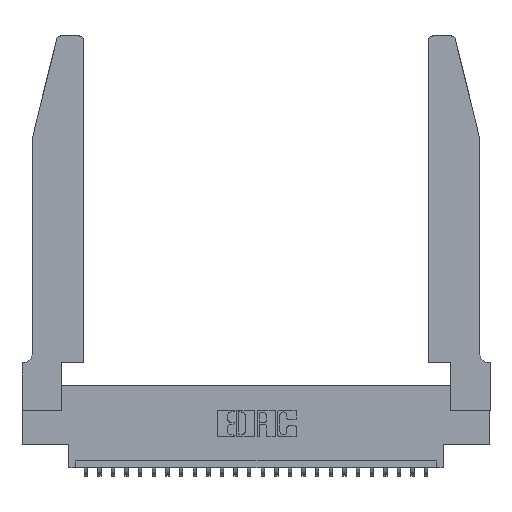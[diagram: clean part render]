
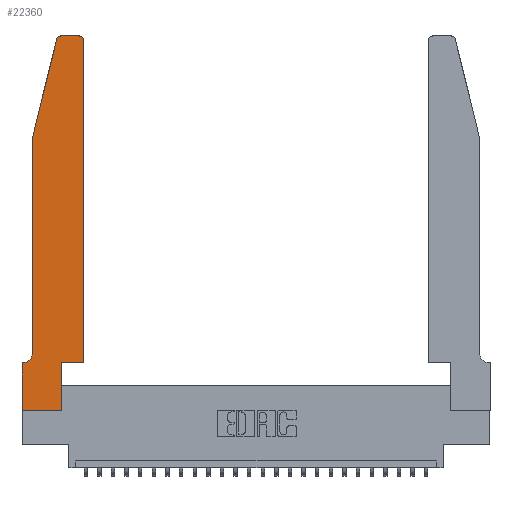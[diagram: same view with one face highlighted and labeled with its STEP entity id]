
A CAD part, top view. The second image highlights one B-rep face of the part: STEP entity #22360.
In plain terms, the highlighted planar face has unit normal (0, 0, 1).
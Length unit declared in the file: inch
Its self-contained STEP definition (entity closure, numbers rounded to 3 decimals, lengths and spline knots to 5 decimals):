
#318 = VERTEX_POINT ( 'NONE', #5157 ) ;
#480 = EDGE_CURVE ( 'NONE', #1135, #4920, #22333, .T. ) ;
#622 = DIRECTION ( 'NONE',  ( 0., 0., 1. ) ) ;
#647 = DIRECTION ( 'NONE',  ( 1., 0., 0. ) ) ;
#790 = VERTEX_POINT ( 'NONE', #2630 ) ;
#998 = VERTEX_POINT ( 'NONE', #18173 ) ;
#1016 = CIRCLE ( 'NONE', #6635, 0.07 ) ;
#1135 = VERTEX_POINT ( 'NONE', #14024 ) ;
#1157 = CARTESIAN_POINT ( 'NONE',  ( 0.0755, 2., 0.37 ) ) ;
#1340 = CARTESIAN_POINT ( 'NONE',  ( 0., 0., 0.37 ) ) ;
#2153 = LINE ( 'NONE', #1157, #8272 ) ;
#2320 = CARTESIAN_POINT ( 'NONE',  ( 0.4505, 0.35, 0.37 ) ) ;
#2576 = VECTOR ( 'NONE', #7749, 39.37008 ) ;
#2629 = LINE ( 'NONE', #14232, #23256 ) ;
#2630 = CARTESIAN_POINT ( 'NONE',  ( 0.0755, 0.42, 0.37 ) ) ;
#3535 = DIRECTION ( 'NONE',  ( 1., 0., 0. ) ) ;
#3636 = CARTESIAN_POINT ( 'NONE',  ( 0.2865, 0.35, 0.37 ) ) ;
#4067 = CARTESIAN_POINT ( 'NONE',  ( 0.0755, 2., 0.37 ) ) ;
#4335 = CARTESIAN_POINT ( 'NONE',  ( 0.2865, 0.35, 0.37 ) ) ;
#4726 = AXIS2_PLACEMENT_3D ( 'NONE', #23396, #622, #15299 ) ;
#4920 = VERTEX_POINT ( 'NONE', #17400 ) ;
#4993 = AXIS2_PLACEMENT_3D ( 'NONE', #7697, #9684, #3535 ) ;
#5065 = CARTESIAN_POINT ( 'NONE',  ( 0.0755, 2., 0.37 ) ) ;
#5157 = CARTESIAN_POINT ( 'NONE',  ( 0.284, 2.75, 0.37 ) ) ;
#5229 = EDGE_CURVE ( 'NONE', #998, #10294, #14947, .T. ) ;
#5653 = CARTESIAN_POINT ( 'NONE',  ( 0.2605, 2.75, 0.37 ) ) ;
#5878 = VERTEX_POINT ( 'NONE', #10979 ) ;
#6230 = AXIS2_PLACEMENT_3D ( 'NONE', #15417, #9199, #647 ) ;
#6256 = DIRECTION ( 'NONE',  ( 0., 1., 0. ) ) ;
#6635 = AXIS2_PLACEMENT_3D ( 'NONE', #18377, #10430, #12156 ) ;
#7697 = CARTESIAN_POINT ( 'NONE',  ( 0.4205, 2.72, 0.37 ) ) ;
#7749 = DIRECTION ( 'NONE',  ( -1., 0., 0. ) ) ;
#8272 = VECTOR ( 'NONE', #19018, 39.37008 ) ;
#8887 = CARTESIAN_POINT ( 'NONE',  ( 0.4505, 0.35, 0.37 ) ) ;
#8955 = VECTOR ( 'NONE', #6256, 39.37008 ) ;
#8995 = VECTOR ( 'NONE', #10202, 39.37008 ) ;
#9176 = PLANE ( 'NONE',  #4726 ) ;
#9195 = ORIENTED_EDGE ( 'NONE', *, *, #9558, .T. ) ;
#9199 = DIRECTION ( 'NONE',  ( 0., 0., 1. ) ) ;
#9322 = EDGE_CURVE ( 'NONE', #24941, #790, #2153, .T. ) ;
#9558 = EDGE_CURVE ( 'NONE', #9641, #13519, #26022, .T. ) ;
#9584 = ORIENTED_EDGE ( 'NONE', *, *, #480, .T. ) ;
#9641 = VERTEX_POINT ( 'NONE', #8887 ) ;
#9684 = DIRECTION ( 'NONE',  ( 0., 0., 1. ) ) ;
#9736 = ORIENTED_EDGE ( 'NONE', *, *, #17080, .T. ) ;
#9824 = VERTEX_POINT ( 'NONE', #13963 ) ;
#10073 = VERTEX_POINT ( 'NONE', #24346 ) ;
#10202 = DIRECTION ( 'NONE',  ( -0.239, -0.971, 0. ) ) ;
#10294 = VERTEX_POINT ( 'NONE', #4335 ) ;
#10430 = DIRECTION ( 'NONE',  ( 0., 0., -1. ) ) ;
#10976 = ORIENTED_EDGE ( 'NONE', *, *, #9322, .T. ) ;
#10979 = CARTESIAN_POINT ( 'NONE',  ( 0.4205, 2.75, 0.37 ) ) ;
#11011 = EDGE_CURVE ( 'NONE', #318, #10073, #23031, .T. ) ;
#11467 = DIRECTION ( 'NONE',  ( -1., 0., 0. ) ) ;
#11927 = DIRECTION ( 'NONE',  ( 0., 1., 0. ) ) ;
#12156 = DIRECTION ( 'NONE',  ( -1., 0., 0. ) ) ;
#12708 = EDGE_LOOP ( 'NONE', ( #9736, #14840, #15039, #10976, #24352, #9584, #16320, #15497, #25948, #16778, #9195, #26026 ) ) ;
#13519 = VERTEX_POINT ( 'NONE', #24000 ) ;
#13668 = LINE ( 'NONE', #1340, #15914 ) ;
#13963 = CARTESIAN_POINT ( 'NONE',  ( 0., 0., 0.37 ) ) ;
#14024 = CARTESIAN_POINT ( 'NONE',  ( 0.0055, 0.35, 0.37 ) ) ;
#14232 = CARTESIAN_POINT ( 'NONE',  ( 0.4505, 0.35, 0.37 ) ) ;
#14840 = ORIENTED_EDGE ( 'NONE', *, *, #11011, .T. ) ;
#14947 = LINE ( 'NONE', #3636, #19771 ) ;
#15039 = ORIENTED_EDGE ( 'NONE', *, *, #23353, .T. ) ;
#15143 = LINE ( 'NONE', #5653, #2576 ) ;
#15299 = DIRECTION ( 'NONE',  ( 1., 0., 0. ) ) ;
#15417 = CARTESIAN_POINT ( 'NONE',  ( 0.284, 2.72, 0.37 ) ) ;
#15461 = LINE ( 'NONE', #4067, #8995 ) ;
#15497 = ORIENTED_EDGE ( 'NONE', *, *, #20556, .T. ) ;
#15914 = VECTOR ( 'NONE', #17654, 39.37008 ) ;
#16042 = CARTESIAN_POINT ( 'NONE',  ( 0., 0., 0.37 ) ) ;
#16320 = ORIENTED_EDGE ( 'NONE', *, *, #23799, .T. ) ;
#16494 = DIRECTION ( 'NONE',  ( 1., 0., 0. ) ) ;
#16778 = ORIENTED_EDGE ( 'NONE', *, *, #22070, .T. ) ;
#17080 = EDGE_CURVE ( 'NONE', #5878, #318, #15143, .T. ) ;
#17400 = CARTESIAN_POINT ( 'NONE',  ( 0., 0.35, 0.37 ) ) ;
#17654 = DIRECTION ( 'NONE',  ( 1., 0., 0. ) ) ;
#17754 = FACE_OUTER_BOUND ( 'NONE', #12708, .T. ) ;
#18004 = EDGE_CURVE ( 'NONE', #13519, #5878, #25080, .T. ) ;
#18173 = CARTESIAN_POINT ( 'NONE',  ( 0.2865, 0., 0.37 ) ) ;
#18377 = CARTESIAN_POINT ( 'NONE',  ( 0.0055, 0.42, 0.37 ) ) ;
#19018 = DIRECTION ( 'NONE',  ( 0., -1., 0. ) ) ;
#19679 = CARTESIAN_POINT ( 'NONE',  ( 0.0755, 0.35, 0.37 ) ) ;
#19771 = VECTOR ( 'NONE', #11927, 39.37008 ) ;
#20556 = EDGE_CURVE ( 'NONE', #9824, #998, #13668, .T. ) ;
#22070 = EDGE_CURVE ( 'NONE', #10294, #9641, #2629, .T. ) ;
#22082 = DIRECTION ( 'NONE',  ( 0., -1., 0. ) ) ;
#22136 = EDGE_CURVE ( 'NONE', #790, #1135, #1016, .T. ) ;
#22333 = LINE ( 'NONE', #19679, #25229 ) ;
#22360 = ADVANCED_FACE ( 'NONE', ( #17754 ), #9176, .T. ) ;
#23031 = CIRCLE ( 'NONE', #6230, 0.03 ) ;
#23256 = VECTOR ( 'NONE', #16494, 39.37008 ) ;
#23353 = EDGE_CURVE ( 'NONE', #10073, #24941, #15461, .T. ) ;
#23396 = CARTESIAN_POINT ( 'NONE',  ( 0., 0.35, 0.37 ) ) ;
#23463 = LINE ( 'NONE', #16042, #24753 ) ;
#23799 = EDGE_CURVE ( 'NONE', #4920, #9824, #23463, .T. ) ;
#24000 = CARTESIAN_POINT ( 'NONE',  ( 0.4505, 2.72, 0.37 ) ) ;
#24346 = CARTESIAN_POINT ( 'NONE',  ( 0.25487, 2.72718, 0.37 ) ) ;
#24352 = ORIENTED_EDGE ( 'NONE', *, *, #22136, .T. ) ;
#24753 = VECTOR ( 'NONE', #22082, 39.37008 ) ;
#24941 = VERTEX_POINT ( 'NONE', #5065 ) ;
#25080 = CIRCLE ( 'NONE', #4993, 0.03 ) ;
#25229 = VECTOR ( 'NONE', #11467, 39.37008 ) ;
#25948 = ORIENTED_EDGE ( 'NONE', *, *, #5229, .T. ) ;
#26022 = LINE ( 'NONE', #2320, #8955 ) ;
#26026 = ORIENTED_EDGE ( 'NONE', *, *, #18004, .T. ) ;
